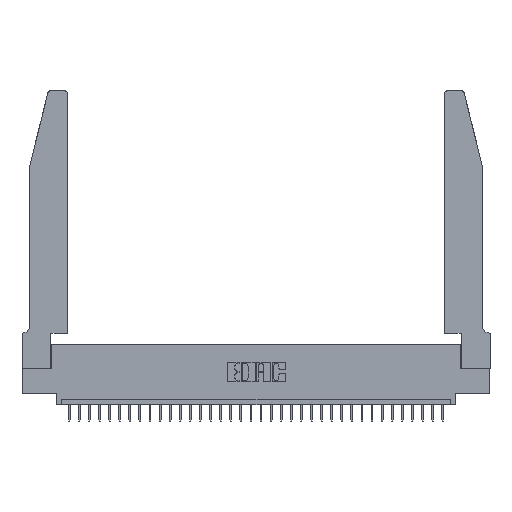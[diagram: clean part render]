
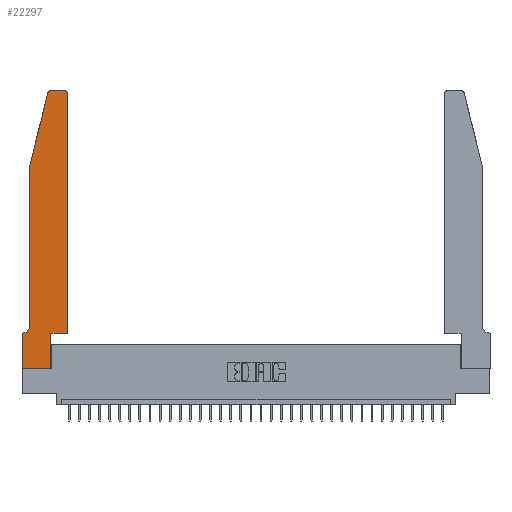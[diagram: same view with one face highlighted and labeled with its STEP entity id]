
A CAD part, top view. The second image highlights one B-rep face of the part: STEP entity #22297.
In plain terms, the highlighted planar face has unit normal (0, 0, 1).
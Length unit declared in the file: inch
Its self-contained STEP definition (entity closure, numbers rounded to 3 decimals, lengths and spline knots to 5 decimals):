
#3 = EDGE_CURVE ( 'NONE', #11022, #23255, #17080, .T. ) ;
#656 = LINE ( 'NONE', #24226, #21709 ) ;
#1768 = LINE ( 'NONE', #20942, #23224 ) ;
#1900 = CIRCLE ( 'NONE', #7906, 0.07 ) ;
#2078 = CARTESIAN_POINT ( 'NONE',  ( 0., 0.35, 0.37 ) ) ;
#2232 = EDGE_CURVE ( 'NONE', #11687, #11022, #5066, .T. ) ;
#2288 = VECTOR ( 'NONE', #19639, 39.37008 ) ;
#2583 = DIRECTION ( 'NONE',  ( -1., 0., 0. ) ) ;
#2589 = VERTEX_POINT ( 'NONE', #30125 ) ;
#2745 = ORIENTED_EDGE ( 'NONE', *, *, #24799, .T. ) ;
#3015 = DIRECTION ( 'NONE',  ( 0., -1., 0. ) ) ;
#4520 = VERTEX_POINT ( 'NONE', #31419 ) ;
#4846 = CIRCLE ( 'NONE', #33457, 0.03 ) ;
#4990 = DIRECTION ( 'NONE',  ( -1., 0., 0. ) ) ;
#5066 = LINE ( 'NONE', #14206, #11602 ) ;
#5268 = EDGE_CURVE ( 'NONE', #12715, #4520, #656, .T. ) ;
#5830 = VECTOR ( 'NONE', #28572, 39.37008 ) ;
#5937 = EDGE_CURVE ( 'NONE', #22898, #22834, #30295, .T. ) ;
#6537 = EDGE_LOOP ( 'NONE', ( #31860, #25993, #29048, #30248, #26869, #21140, #19334, #21671, #15368, #20011, #2745, #27811 ) ) ;
#7261 = EDGE_CURVE ( 'NONE', #28747, #33908, #22099, .T. ) ;
#7310 = DIRECTION ( 'NONE',  ( -1., 0., 0. ) ) ;
#7341 = DIRECTION ( 'NONE',  ( 1., 0., 0. ) ) ;
#7906 = AXIS2_PLACEMENT_3D ( 'NONE', #26155, #33644, #4990 ) ;
#8389 = FACE_OUTER_BOUND ( 'NONE', #6537, .T. ) ;
#9068 = DIRECTION ( 'NONE',  ( 0., -1., 0. ) ) ;
#9127 = EDGE_CURVE ( 'NONE', #30669, #31401, #4846, .T. ) ;
#9246 = CARTESIAN_POINT ( 'NONE',  ( 0.4505, 2.72, 0.37 ) ) ;
#9276 = VECTOR ( 'NONE', #7341, 39.37008 ) ;
#9749 = EDGE_CURVE ( 'NONE', #4520, #2589, #1900, .T. ) ;
#9809 = CARTESIAN_POINT ( 'NONE',  ( 0.284, 2.75, 0.37 ) ) ;
#10043 = CARTESIAN_POINT ( 'NONE',  ( 0.0755, 0.35, 0.37 ) ) ;
#10053 = AXIS2_PLACEMENT_3D ( 'NONE', #15523, #26021, #28693 ) ;
#11022 = VERTEX_POINT ( 'NONE', #23358 ) ;
#11602 = VECTOR ( 'NONE', #9068, 39.37008 ) ;
#11687 = VERTEX_POINT ( 'NONE', #2078 ) ;
#11737 = CARTESIAN_POINT ( 'NONE',  ( 0.0755, 2., 0.37 ) ) ;
#12651 = CARTESIAN_POINT ( 'NONE',  ( 0.2865, 0.35, 0.37 ) ) ;
#12715 = VERTEX_POINT ( 'NONE', #11737 ) ;
#13580 = CARTESIAN_POINT ( 'NONE',  ( 0.0755, 2., 0.37 ) ) ;
#13660 = CARTESIAN_POINT ( 'NONE',  ( 0.4505, 0.35, 0.37 ) ) ;
#13857 = VECTOR ( 'NONE', #31932, 39.37008 ) ;
#14206 = CARTESIAN_POINT ( 'NONE',  ( 0., 0., 0.37 ) ) ;
#15368 = ORIENTED_EDGE ( 'NONE', *, *, #27669, .T. ) ;
#15523 = CARTESIAN_POINT ( 'NONE',  ( 0.4205, 2.72, 0.37 ) ) ;
#16231 = DIRECTION ( 'NONE',  ( 0., 1., 0. ) ) ;
#16940 = CARTESIAN_POINT ( 'NONE',  ( 0., 0., 0.37 ) ) ;
#17080 = LINE ( 'NONE', #16940, #2288 ) ;
#19236 = CARTESIAN_POINT ( 'NONE',  ( 0.2865, 0.35, 0.37 ) ) ;
#19334 = ORIENTED_EDGE ( 'NONE', *, *, #2232, .T. ) ;
#19639 = DIRECTION ( 'NONE',  ( 1., 0., 0. ) ) ;
#20011 = ORIENTED_EDGE ( 'NONE', *, *, #5937, .T. ) ;
#20523 = LINE ( 'NONE', #13580, #13857 ) ;
#20942 = CARTESIAN_POINT ( 'NONE',  ( 0.2605, 2.75, 0.37 ) ) ;
#21140 = ORIENTED_EDGE ( 'NONE', *, *, #31464, .T. ) ;
#21270 = VECTOR ( 'NONE', #7310, 39.37008 ) ;
#21671 = ORIENTED_EDGE ( 'NONE', *, *, #3, .T. ) ;
#21709 = VECTOR ( 'NONE', #3015, 39.37008 ) ;
#22099 = CIRCLE ( 'NONE', #10053, 0.03 ) ;
#22297 = ADVANCED_FACE ( 'NONE', ( #8389 ), #23818, .T. ) ;
#22834 = VERTEX_POINT ( 'NONE', #13660 ) ;
#22898 = VERTEX_POINT ( 'NONE', #19236 ) ;
#23118 = CARTESIAN_POINT ( 'NONE',  ( 0.4505, 0.35, 0.37 ) ) ;
#23224 = VECTOR ( 'NONE', #2583, 39.37008 ) ;
#23255 = VERTEX_POINT ( 'NONE', #30950 ) ;
#23358 = CARTESIAN_POINT ( 'NONE',  ( 0., 0., 0.37 ) ) ;
#23818 = PLANE ( 'NONE',  #25840 ) ;
#23928 = DIRECTION ( 'NONE',  ( 1., 0., 0. ) ) ;
#24046 = CARTESIAN_POINT ( 'NONE',  ( 0.4205, 2.75, 0.37 ) ) ;
#24226 = CARTESIAN_POINT ( 'NONE',  ( 0.0755, 2., 0.37 ) ) ;
#24264 = LINE ( 'NONE', #26721, #34126 ) ;
#24799 = EDGE_CURVE ( 'NONE', #22834, #28747, #24264, .T. ) ;
#24949 = LINE ( 'NONE', #10043, #21270 ) ;
#25840 = AXIS2_PLACEMENT_3D ( 'NONE', #31966, #26439, #23928 ) ;
#25993 = ORIENTED_EDGE ( 'NONE', *, *, #9127, .T. ) ;
#26021 = DIRECTION ( 'NONE',  ( 0., 0., 1. ) ) ;
#26155 = CARTESIAN_POINT ( 'NONE',  ( 0.0055, 0.42, 0.37 ) ) ;
#26439 = DIRECTION ( 'NONE',  ( 0., 0., 1. ) ) ;
#26721 = CARTESIAN_POINT ( 'NONE',  ( 0.4505, 0.35, 0.37 ) ) ;
#26830 = LINE ( 'NONE', #12651, #5830 ) ;
#26869 = ORIENTED_EDGE ( 'NONE', *, *, #9749, .T. ) ;
#27669 = EDGE_CURVE ( 'NONE', #23255, #22898, #26830, .T. ) ;
#27811 = ORIENTED_EDGE ( 'NONE', *, *, #7261, .T. ) ;
#28572 = DIRECTION ( 'NONE',  ( 0., 1., 0. ) ) ;
#28670 = DIRECTION ( 'NONE',  ( 1., 0., 0. ) ) ;
#28693 = DIRECTION ( 'NONE',  ( 1., 0., 0. ) ) ;
#28747 = VERTEX_POINT ( 'NONE', #9246 ) ;
#29048 = ORIENTED_EDGE ( 'NONE', *, *, #30479, .T. ) ;
#30125 = CARTESIAN_POINT ( 'NONE',  ( 0.0055, 0.35, 0.37 ) ) ;
#30248 = ORIENTED_EDGE ( 'NONE', *, *, #5268, .T. ) ;
#30295 = LINE ( 'NONE', #23118, #9276 ) ;
#30479 = EDGE_CURVE ( 'NONE', #31401, #12715, #20523, .T. ) ;
#30669 = VERTEX_POINT ( 'NONE', #9809 ) ;
#30950 = CARTESIAN_POINT ( 'NONE',  ( 0.2865, 0., 0.37 ) ) ;
#31401 = VERTEX_POINT ( 'NONE', #31604 ) ;
#31419 = CARTESIAN_POINT ( 'NONE',  ( 0.0755, 0.42, 0.37 ) ) ;
#31464 = EDGE_CURVE ( 'NONE', #2589, #11687, #24949, .T. ) ;
#31604 = CARTESIAN_POINT ( 'NONE',  ( 0.25487, 2.72718, 0.37 ) ) ;
#31860 = ORIENTED_EDGE ( 'NONE', *, *, #32809, .T. ) ;
#31932 = DIRECTION ( 'NONE',  ( -0.239, -0.971, 0. ) ) ;
#31966 = CARTESIAN_POINT ( 'NONE',  ( 0., 0.35, 0.37 ) ) ;
#32809 = EDGE_CURVE ( 'NONE', #33908, #30669, #1768, .T. ) ;
#33457 = AXIS2_PLACEMENT_3D ( 'NONE', #33826, #33937, #28670 ) ;
#33644 = DIRECTION ( 'NONE',  ( 0., 0., -1. ) ) ;
#33826 = CARTESIAN_POINT ( 'NONE',  ( 0.284, 2.72, 0.37 ) ) ;
#33908 = VERTEX_POINT ( 'NONE', #24046 ) ;
#33937 = DIRECTION ( 'NONE',  ( 0., 0., 1. ) ) ;
#34126 = VECTOR ( 'NONE', #16231, 39.37008 ) ;
